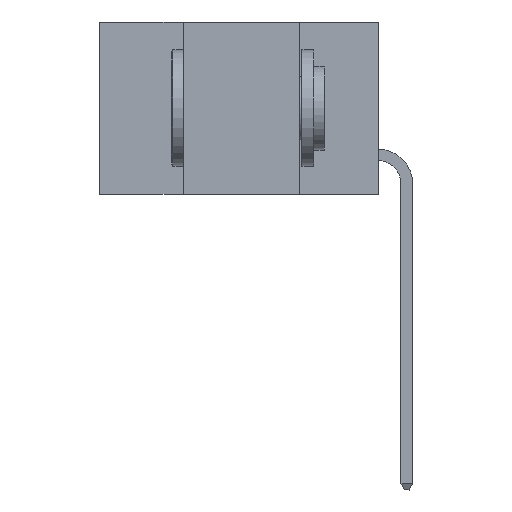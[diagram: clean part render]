
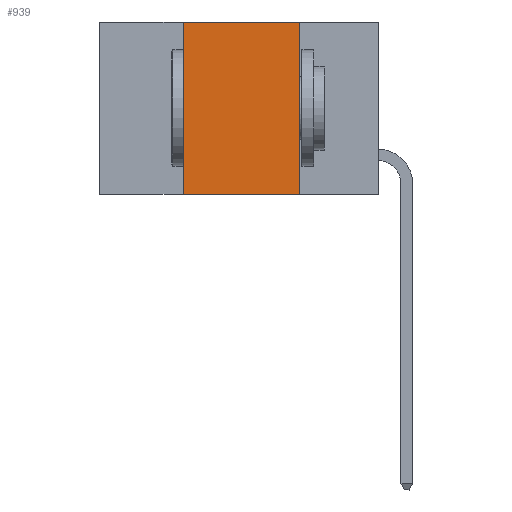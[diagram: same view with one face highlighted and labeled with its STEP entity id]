
A CAD part, left-side view. The second image highlights one B-rep face of the part: STEP entity #939.
In plain terms, the highlighted planar face has unit normal (-1, 0, 0).
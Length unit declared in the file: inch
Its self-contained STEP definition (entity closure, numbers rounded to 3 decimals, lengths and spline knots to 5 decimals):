
#939 = ADVANCED_FACE ( 'NONE', ( #2222 ), #12741, .F. ) ;
#1792 = ORIENTED_EDGE ( 'NONE', *, *, #11522, .F. ) ;
#1814 = CARTESIAN_POINT ( 'NONE',  ( 0., 0.6, -0.37 ) ) ;
#2087 = LINE ( 'NONE', #16698, #5630 ) ;
#2222 = FACE_OUTER_BOUND ( 'NONE', #12382, .T. ) ;
#3568 = AXIS2_PLACEMENT_3D ( 'NONE', #18008, #14896, #14739 ) ;
#3815 = CARTESIAN_POINT ( 'NONE',  ( 0., 0.6, 0. ) ) ;
#3897 = DIRECTION ( 'NONE',  ( 0., 0., -1. ) ) ;
#4091 = EDGE_CURVE ( 'NONE', #10345, #15591, #16247, .T. ) ;
#4785 = LINE ( 'NONE', #1814, #16063 ) ;
#4986 = DIRECTION ( 'NONE',  ( 0., 0., 1. ) ) ;
#5399 = CARTESIAN_POINT ( 'NONE',  ( 0., 0.17, 0. ) ) ;
#5630 = VECTOR ( 'NONE', #4986, 39.37008 ) ;
#6516 = CARTESIAN_POINT ( 'NONE',  ( 0., 0.17, 0. ) ) ;
#7541 = VERTEX_POINT ( 'NONE', #15252 ) ;
#7621 = VECTOR ( 'NONE', #3897, 39.37008 ) ;
#8078 = LINE ( 'NONE', #5399, #7621 ) ;
#9527 = EDGE_CURVE ( 'NONE', #16593, #7541, #4785, .T. ) ;
#9732 = ORIENTED_EDGE ( 'NONE', *, *, #9527, .T. ) ;
#10345 = VERTEX_POINT ( 'NONE', #12628 ) ;
#10965 = DIRECTION ( 'NONE',  ( 0., -1., 0. ) ) ;
#11522 = EDGE_CURVE ( 'NONE', #16593, #10345, #2087, .T. ) ;
#12297 = ORIENTED_EDGE ( 'NONE', *, *, #14474, .F. ) ;
#12382 = EDGE_LOOP ( 'NONE', ( #12297, #13206, #1792, #9732 ) ) ;
#12628 = CARTESIAN_POINT ( 'NONE',  ( 0., 0.42, 0. ) ) ;
#12741 = PLANE ( 'NONE',  #3568 ) ;
#13206 = ORIENTED_EDGE ( 'NONE', *, *, #4091, .F. ) ;
#13331 = CARTESIAN_POINT ( 'NONE',  ( 0., 0.42, -0.37 ) ) ;
#13726 = DIRECTION ( 'NONE',  ( 0., -1., 0. ) ) ;
#14474 = EDGE_CURVE ( 'NONE', #15591, #7541, #8078, .T. ) ;
#14739 = DIRECTION ( 'NONE',  ( 0., 0., -1. ) ) ;
#14896 = DIRECTION ( 'NONE',  ( 1., 0., 0. ) ) ;
#15252 = CARTESIAN_POINT ( 'NONE',  ( 0., 0.17, -0.37 ) ) ;
#15591 = VERTEX_POINT ( 'NONE', #6516 ) ;
#15784 = VECTOR ( 'NONE', #10965, 39.37008 ) ;
#16063 = VECTOR ( 'NONE', #13726, 39.37008 ) ;
#16247 = LINE ( 'NONE', #3815, #15784 ) ;
#16593 = VERTEX_POINT ( 'NONE', #13331 ) ;
#16698 = CARTESIAN_POINT ( 'NONE',  ( 0., 0.42, 0. ) ) ;
#18008 = CARTESIAN_POINT ( 'NONE',  ( 0., 0.6, 0. ) ) ;
